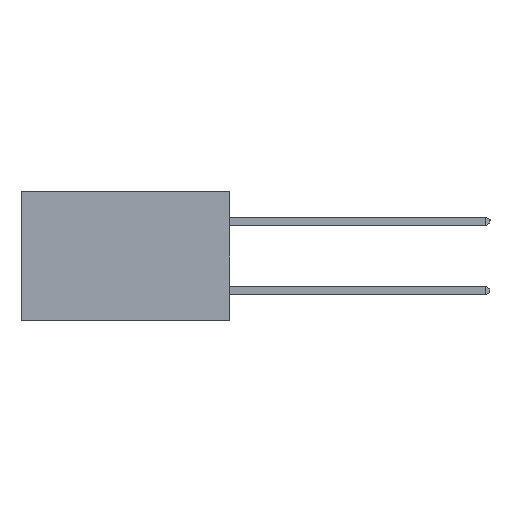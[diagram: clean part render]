
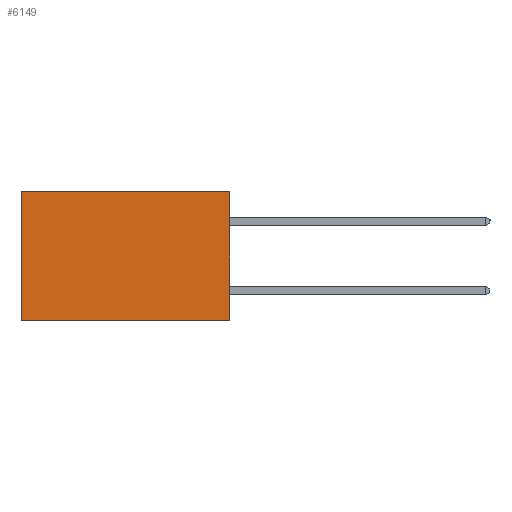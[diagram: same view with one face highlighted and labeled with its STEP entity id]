
A CAD part, left-side view. The second image highlights one B-rep face of the part: STEP entity #6149.
In plain terms, the highlighted planar face has unit normal (-1, 0, 0).
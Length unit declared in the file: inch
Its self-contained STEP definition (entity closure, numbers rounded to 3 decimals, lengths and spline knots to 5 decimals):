
#415 = CARTESIAN_POINT ( 'NONE',  ( 0.2615, 0.6, -0.37 ) ) ;
#722 = DIRECTION ( 'NONE',  ( 0., 1., 0. ) ) ;
#788 = ORIENTED_EDGE ( 'NONE', *, *, #2063, .T. ) ;
#822 = VERTEX_POINT ( 'NONE', #8668 ) ;
#975 = EDGE_CURVE ( 'NONE', #2297, #7357, #1956, .T. ) ;
#1062 = ORIENTED_EDGE ( 'NONE', *, *, #9099, .T. ) ;
#1072 = CARTESIAN_POINT ( 'NONE',  ( 0.2615, 0., -0.37 ) ) ;
#1239 = VECTOR ( 'NONE', #6365, 39.37008 ) ;
#1956 = LINE ( 'NONE', #10776, #1239 ) ;
#1980 = VECTOR ( 'NONE', #3942, 39.37008 ) ;
#2063 = EDGE_CURVE ( 'NONE', #822, #7188, #7255, .T. ) ;
#2242 = ORIENTED_EDGE ( 'NONE', *, *, #975, .F. ) ;
#2297 = VERTEX_POINT ( 'NONE', #4724 ) ;
#2577 = EDGE_LOOP ( 'NONE', ( #788, #7847, #2242, #1062 ) ) ;
#2634 = FACE_OUTER_BOUND ( 'NONE', #2577, .T. ) ;
#2819 = CARTESIAN_POINT ( 'NONE',  ( 0.2615, 0., 0. ) ) ;
#3225 = CARTESIAN_POINT ( 'NONE',  ( 0.2615, 0.6, -0.37 ) ) ;
#3386 = DIRECTION ( 'NONE',  ( 0., 1., 0. ) ) ;
#3942 = DIRECTION ( 'NONE',  ( 0., 0., -1. ) ) ;
#4719 = VECTOR ( 'NONE', #3386, 39.37008 ) ;
#4724 = CARTESIAN_POINT ( 'NONE',  ( 0.2615, 0., 0. ) ) ;
#5741 = CARTESIAN_POINT ( 'NONE',  ( 0.2615, 0., -0.37 ) ) ;
#6133 = DIRECTION ( 'NONE',  ( 1., 0., 0. ) ) ;
#6149 = ADVANCED_FACE ( 'NONE', ( #2634 ), #8821, .F. ) ;
#6365 = DIRECTION ( 'NONE',  ( 0., 0., -1. ) ) ;
#6993 = CARTESIAN_POINT ( 'NONE',  ( 0.2615, 0., -0.37 ) ) ;
#7188 = VERTEX_POINT ( 'NONE', #3225 ) ;
#7255 = LINE ( 'NONE', #415, #1980 ) ;
#7357 = VERTEX_POINT ( 'NONE', #6993 ) ;
#7450 = LINE ( 'NONE', #5741, #10414 ) ;
#7800 = AXIS2_PLACEMENT_3D ( 'NONE', #1072, #6133, #9791 ) ;
#7847 = ORIENTED_EDGE ( 'NONE', *, *, #11169, .F. ) ;
#8668 = CARTESIAN_POINT ( 'NONE',  ( 0.2615, 0.6, 0. ) ) ;
#8821 = PLANE ( 'NONE',  #7800 ) ;
#9099 = EDGE_CURVE ( 'NONE', #2297, #822, #10674, .T. ) ;
#9791 = DIRECTION ( 'NONE',  ( 0., 0., -1. ) ) ;
#10414 = VECTOR ( 'NONE', #722, 39.37008 ) ;
#10674 = LINE ( 'NONE', #2819, #4719 ) ;
#10776 = CARTESIAN_POINT ( 'NONE',  ( 0.2615, 0., -0.37 ) ) ;
#11169 = EDGE_CURVE ( 'NONE', #7357, #7188, #7450, .T. ) ;
